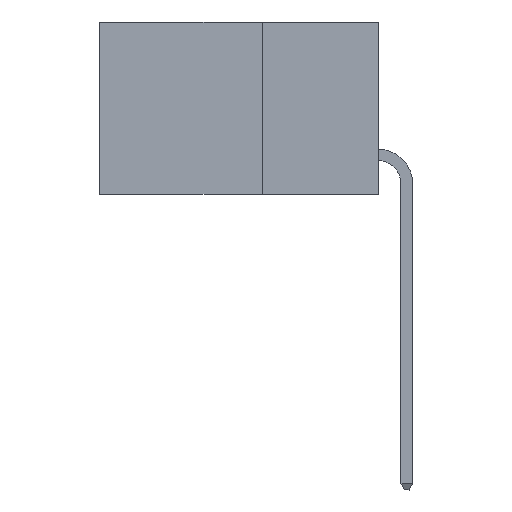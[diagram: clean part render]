
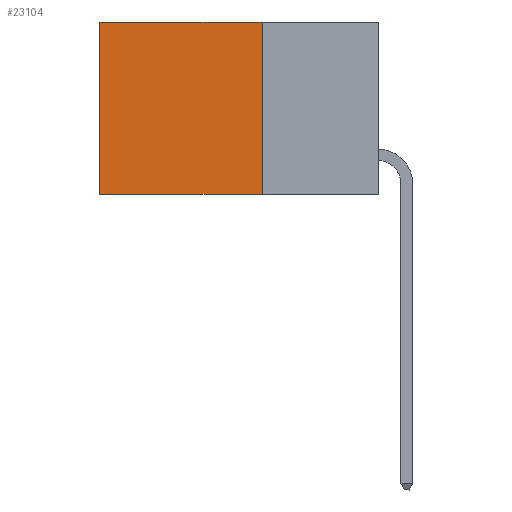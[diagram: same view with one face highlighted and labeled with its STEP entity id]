
A CAD part, left-side view. The second image highlights one B-rep face of the part: STEP entity #23104.
In plain terms, the highlighted planar face has unit normal (-1, 0, 0).
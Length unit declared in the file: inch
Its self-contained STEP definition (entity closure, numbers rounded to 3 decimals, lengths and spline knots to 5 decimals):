
#351 = CARTESIAN_POINT ( 'NONE',  ( 0.2615, 0.25, -0.37 ) ) ;
#516 = DIRECTION ( 'NONE',  ( 0., 0., -1. ) ) ;
#1807 = LINE ( 'NONE', #21731, #17619 ) ;
#2196 = DIRECTION ( 'NONE',  ( 0., 1., 0. ) ) ;
#2201 = PLANE ( 'NONE',  #21129 ) ;
#6842 = CARTESIAN_POINT ( 'NONE',  ( 0.2615, 0.25, -0.37 ) ) ;
#7715 = CARTESIAN_POINT ( 'NONE',  ( 0.2615, 0.6, -0.37 ) ) ;
#7725 = VERTEX_POINT ( 'NONE', #19320 ) ;
#8194 = LINE ( 'NONE', #351, #23001 ) ;
#10265 = EDGE_CURVE ( 'NONE', #10343, #13492, #19279, .T. ) ;
#10343 = VERTEX_POINT ( 'NONE', #14050 ) ;
#10543 = VERTEX_POINT ( 'NONE', #20414 ) ;
#11182 = EDGE_CURVE ( 'NONE', #7725, #10343, #1807, .T. ) ;
#11666 = ORIENTED_EDGE ( 'NONE', *, *, #10265, .T. ) ;
#12058 = FACE_OUTER_BOUND ( 'NONE', #24516, .T. ) ;
#12438 = LINE ( 'NONE', #6842, #17782 ) ;
#13492 = VERTEX_POINT ( 'NONE', #16393 ) ;
#13547 = DIRECTION ( 'NONE',  ( 0., 0., -1. ) ) ;
#13580 = VECTOR ( 'NONE', #13547, 39.37008 ) ;
#14050 = CARTESIAN_POINT ( 'NONE',  ( 0.2615, 0.6, 0. ) ) ;
#16393 = CARTESIAN_POINT ( 'NONE',  ( 0.2615, 0.6, -0.37 ) ) ;
#17417 = EDGE_CURVE ( 'NONE', #10543, #13492, #8194, .T. ) ;
#17479 = ORIENTED_EDGE ( 'NONE', *, *, #18734, .F. ) ;
#17619 = VECTOR ( 'NONE', #2196, 39.37008 ) ;
#17782 = VECTOR ( 'NONE', #516, 39.37008 ) ;
#17863 = ORIENTED_EDGE ( 'NONE', *, *, #17417, .F. ) ;
#18734 = EDGE_CURVE ( 'NONE', #7725, #10543, #12438, .T. ) ;
#19279 = LINE ( 'NONE', #7715, #13580 ) ;
#19320 = CARTESIAN_POINT ( 'NONE',  ( 0.2615, 0.25, 0. ) ) ;
#19647 = DIRECTION ( 'NONE',  ( 0., 1., 0. ) ) ;
#20414 = CARTESIAN_POINT ( 'NONE',  ( 0.2615, 0.25, -0.37 ) ) ;
#20941 = ORIENTED_EDGE ( 'NONE', *, *, #11182, .T. ) ;
#21129 = AXIS2_PLACEMENT_3D ( 'NONE', #23675, #23294, #23415 ) ;
#21731 = CARTESIAN_POINT ( 'NONE',  ( 0.2615, 0.25, 0. ) ) ;
#23001 = VECTOR ( 'NONE', #19647, 39.37008 ) ;
#23104 = ADVANCED_FACE ( 'NONE', ( #12058 ), #2201, .F. ) ;
#23294 = DIRECTION ( 'NONE',  ( 1., 0., 0. ) ) ;
#23415 = DIRECTION ( 'NONE',  ( 0., 0., -1. ) ) ;
#23675 = CARTESIAN_POINT ( 'NONE',  ( 0.2615, 0.25, -0.37 ) ) ;
#24516 = EDGE_LOOP ( 'NONE', ( #11666, #17863, #17479, #20941 ) ) ;
